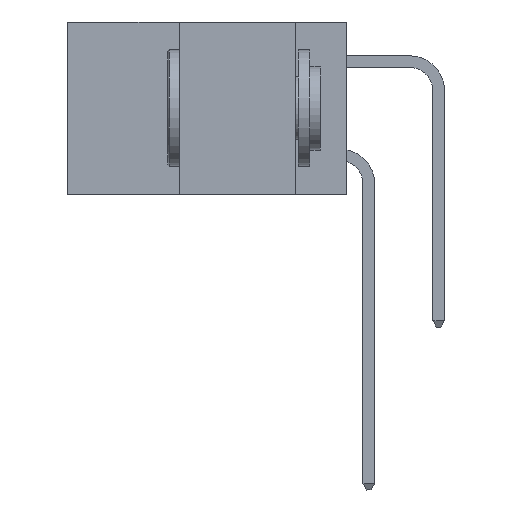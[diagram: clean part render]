
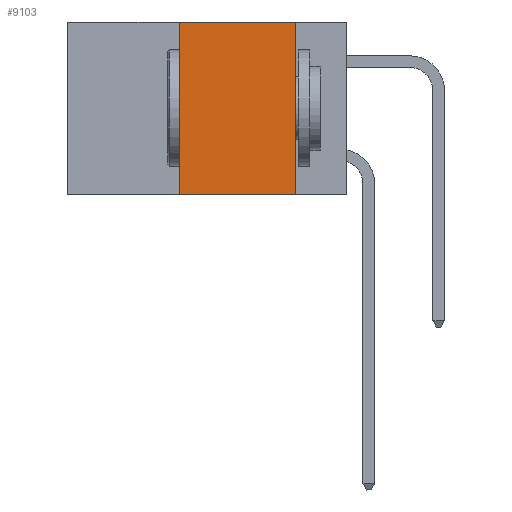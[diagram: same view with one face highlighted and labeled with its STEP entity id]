
A CAD part, left-side view. The second image highlights one B-rep face of the part: STEP entity #9103.
In plain terms, the highlighted planar face has unit normal (-1, 0, 0).
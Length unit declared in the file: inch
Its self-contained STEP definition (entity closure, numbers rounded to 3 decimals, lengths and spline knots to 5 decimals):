
#886 = VERTEX_POINT ( 'NONE', #5229 ) ;
#1116 = CARTESIAN_POINT ( 'NONE',  ( 0., 0.11, -0.37 ) ) ;
#1603 = CARTESIAN_POINT ( 'NONE',  ( 0., 0.36, 0. ) ) ;
#2615 = VERTEX_POINT ( 'NONE', #1603 ) ;
#2675 = CARTESIAN_POINT ( 'NONE',  ( 0., 0.36, 0. ) ) ;
#2745 = LINE ( 'NONE', #12069, #16105 ) ;
#3101 = VERTEX_POINT ( 'NONE', #18492 ) ;
#4416 = VECTOR ( 'NONE', #20512, 39.37008 ) ;
#4660 = EDGE_CURVE ( 'NONE', #3101, #8830, #2745, .T. ) ;
#5108 = EDGE_CURVE ( 'NONE', #886, #2615, #7428, .T. ) ;
#5229 = CARTESIAN_POINT ( 'NONE',  ( 0., 0.36, -0.37 ) ) ;
#5893 = FACE_OUTER_BOUND ( 'NONE', #11256, .T. ) ;
#6467 = LINE ( 'NONE', #10288, #19749 ) ;
#7428 = LINE ( 'NONE', #2675, #12070 ) ;
#7933 = ORIENTED_EDGE ( 'NONE', *, *, #4660, .F. ) ;
#8830 = VERTEX_POINT ( 'NONE', #1116 ) ;
#9103 = ADVANCED_FACE ( 'NONE', ( #5893 ), #19767, .F. ) ;
#9351 = ORIENTED_EDGE ( 'NONE', *, *, #5108, .F. ) ;
#9457 = CARTESIAN_POINT ( 'NONE',  ( 0., 0.6, 0. ) ) ;
#10288 = CARTESIAN_POINT ( 'NONE',  ( 0., 0.6, -0.37 ) ) ;
#11215 = DIRECTION ( 'NONE',  ( 0., 0., -1. ) ) ;
#11227 = EDGE_CURVE ( 'NONE', #2615, #3101, #18225, .T. ) ;
#11256 = EDGE_LOOP ( 'NONE', ( #7933, #19831, #9351, #12602 ) ) ;
#12069 = CARTESIAN_POINT ( 'NONE',  ( 0., 0.11, 0. ) ) ;
#12070 = VECTOR ( 'NONE', #14915, 39.37008 ) ;
#12602 = ORIENTED_EDGE ( 'NONE', *, *, #18726, .T. ) ;
#14915 = DIRECTION ( 'NONE',  ( 0., 0., 1. ) ) ;
#16105 = VECTOR ( 'NONE', #18968, 39.37008 ) ;
#17163 = DIRECTION ( 'NONE',  ( 0., -1., 0. ) ) ;
#18225 = LINE ( 'NONE', #22116, #4416 ) ;
#18492 = CARTESIAN_POINT ( 'NONE',  ( 0., 0.11, 0. ) ) ;
#18726 = EDGE_CURVE ( 'NONE', #886, #8830, #6467, .T. ) ;
#18968 = DIRECTION ( 'NONE',  ( 0., 0., -1. ) ) ;
#19749 = VECTOR ( 'NONE', #17163, 39.37008 ) ;
#19767 = PLANE ( 'NONE',  #21441 ) ;
#19831 = ORIENTED_EDGE ( 'NONE', *, *, #11227, .F. ) ;
#20512 = DIRECTION ( 'NONE',  ( 0., -1., 0. ) ) ;
#21441 = AXIS2_PLACEMENT_3D ( 'NONE', #9457, #21459, #11215 ) ;
#21459 = DIRECTION ( 'NONE',  ( 1., 0., 0. ) ) ;
#22116 = CARTESIAN_POINT ( 'NONE',  ( 0., 0.6, 0. ) ) ;
